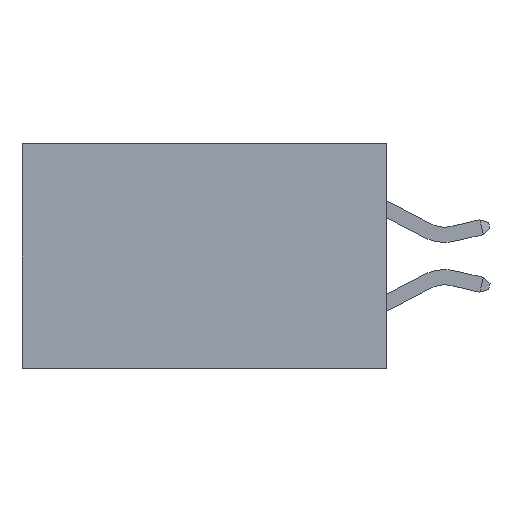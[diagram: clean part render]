
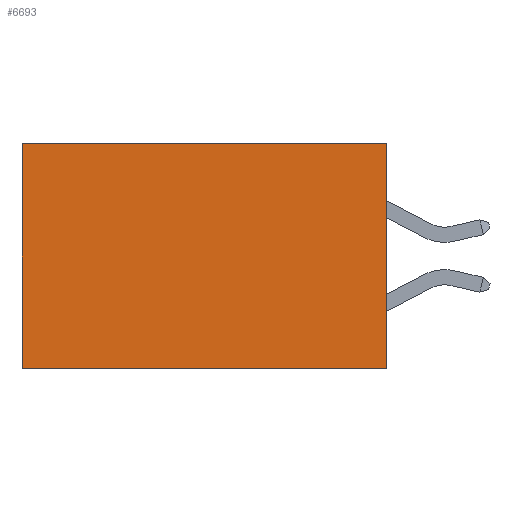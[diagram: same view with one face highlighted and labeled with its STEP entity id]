
A CAD part, left-side view. The second image highlights one B-rep face of the part: STEP entity #6693.
In plain terms, the highlighted planar face has unit normal (-1, 0, 0).
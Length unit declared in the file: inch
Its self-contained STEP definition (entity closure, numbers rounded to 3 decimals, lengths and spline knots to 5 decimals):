
#109 = FACE_OUTER_BOUND ( 'NONE', #6154, .T. ) ;
#470 = VERTEX_POINT ( 'NONE', #8978 ) ;
#1056 = DIRECTION ( 'NONE',  ( 0., 0., -1. ) ) ;
#1280 = VECTOR ( 'NONE', #9792, 39.37008 ) ;
#2631 = CARTESIAN_POINT ( 'NONE',  ( 0.2615, 0., -0.37 ) ) ;
#2989 = ORIENTED_EDGE ( 'NONE', *, *, #7363, .T. ) ;
#3399 = CARTESIAN_POINT ( 'NONE',  ( 0.2615, 0.6, 0. ) ) ;
#3845 = VERTEX_POINT ( 'NONE', #10512 ) ;
#3864 = ORIENTED_EDGE ( 'NONE', *, *, #7961, .F. ) ;
#3961 = LINE ( 'NONE', #4468, #10191 ) ;
#4468 = CARTESIAN_POINT ( 'NONE',  ( 0.2615, 0.6, -0.37 ) ) ;
#4509 = ORIENTED_EDGE ( 'NONE', *, *, #8234, .T. ) ;
#4561 = LINE ( 'NONE', #2631, #8730 ) ;
#4903 = AXIS2_PLACEMENT_3D ( 'NONE', #5568, #6457, #1056 ) ;
#5054 = DIRECTION ( 'NONE',  ( 0., 1., 0. ) ) ;
#5205 = VERTEX_POINT ( 'NONE', #3399 ) ;
#5568 = CARTESIAN_POINT ( 'NONE',  ( 0.2615, 0., -0.37 ) ) ;
#6154 = EDGE_LOOP ( 'NONE', ( #2989, #6476, #3864, #4509 ) ) ;
#6211 = LINE ( 'NONE', #8377, #8372 ) ;
#6349 = LINE ( 'NONE', #6653, #1280 ) ;
#6457 = DIRECTION ( 'NONE',  ( 1., 0., 0. ) ) ;
#6476 = ORIENTED_EDGE ( 'NONE', *, *, #7814, .F. ) ;
#6653 = CARTESIAN_POINT ( 'NONE',  ( 0.2615, 0., 0. ) ) ;
#6693 = ADVANCED_FACE ( 'NONE', ( #109 ), #10385, .F. ) ;
#7363 = EDGE_CURVE ( 'NONE', #5205, #3845, #3961, .T. ) ;
#7814 = EDGE_CURVE ( 'NONE', #470, #3845, #6211, .T. ) ;
#7961 = EDGE_CURVE ( 'NONE', #9536, #470, #4561, .T. ) ;
#8234 = EDGE_CURVE ( 'NONE', #9536, #5205, #6349, .T. ) ;
#8372 = VECTOR ( 'NONE', #5054, 39.37008 ) ;
#8377 = CARTESIAN_POINT ( 'NONE',  ( 0.2615, 0., -0.37 ) ) ;
#8625 = CARTESIAN_POINT ( 'NONE',  ( 0.2615, 0., 0. ) ) ;
#8721 = DIRECTION ( 'NONE',  ( 0., 0., -1. ) ) ;
#8730 = VECTOR ( 'NONE', #10838, 39.37008 ) ;
#8978 = CARTESIAN_POINT ( 'NONE',  ( 0.2615, 0., -0.37 ) ) ;
#9536 = VERTEX_POINT ( 'NONE', #8625 ) ;
#9792 = DIRECTION ( 'NONE',  ( 0., 1., 0. ) ) ;
#10191 = VECTOR ( 'NONE', #8721, 39.37008 ) ;
#10385 = PLANE ( 'NONE',  #4903 ) ;
#10512 = CARTESIAN_POINT ( 'NONE',  ( 0.2615, 0.6, -0.37 ) ) ;
#10838 = DIRECTION ( 'NONE',  ( 0., 0., -1. ) ) ;
